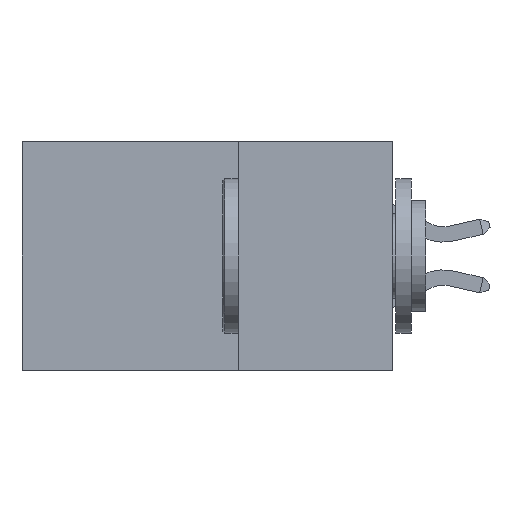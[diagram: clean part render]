
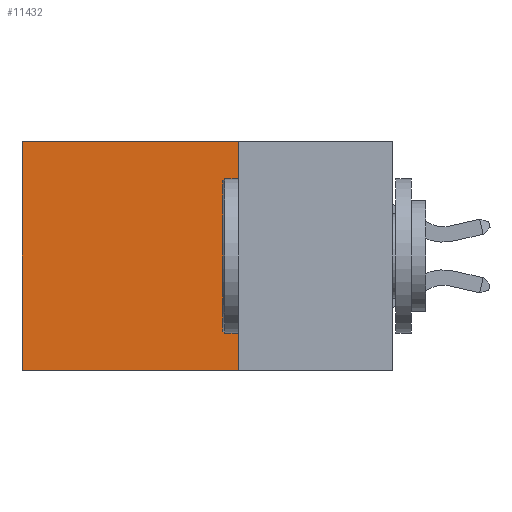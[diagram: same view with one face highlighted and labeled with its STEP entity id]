
A CAD part, left-side view. The second image highlights one B-rep face of the part: STEP entity #11432.
In plain terms, the highlighted planar face has unit normal (-1, 0, 0).
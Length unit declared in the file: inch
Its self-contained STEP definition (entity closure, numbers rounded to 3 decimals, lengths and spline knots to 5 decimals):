
#77 = AXIS2_PLACEMENT_3D ( 'NONE', #11838, #18074, #5435 ) ;
#2755 = VECTOR ( 'NONE', #4926, 39.37008 ) ;
#2768 = CARTESIAN_POINT ( 'NONE',  ( 0.2875, 0.25, -0.37 ) ) ;
#4536 = ORIENTED_EDGE ( 'NONE', *, *, #21344, .F. ) ;
#4926 = DIRECTION ( 'NONE',  ( 0., 0., -1. ) ) ;
#4946 = CARTESIAN_POINT ( 'NONE',  ( 0.2875, 0.6, -0.37 ) ) ;
#5435 = DIRECTION ( 'NONE',  ( 0., 0., -1. ) ) ;
#6113 = VECTOR ( 'NONE', #25194, 39.37008 ) ;
#6768 = LINE ( 'NONE', #23016, #6113 ) ;
#7376 = CARTESIAN_POINT ( 'NONE',  ( 0.2875, 0.25, 0. ) ) ;
#7511 = PLANE ( 'NONE',  #77 ) ;
#8352 = VERTEX_POINT ( 'NONE', #4946 ) ;
#8632 = LINE ( 'NONE', #7376, #19130 ) ;
#8957 = VERTEX_POINT ( 'NONE', #21779 ) ;
#9541 = DIRECTION ( 'NONE',  ( 0., 1., 0. ) ) ;
#11217 = FACE_OUTER_BOUND ( 'NONE', #12395, .T. ) ;
#11432 = ADVANCED_FACE ( 'NONE', ( #11217 ), #7511, .F. ) ;
#11838 = CARTESIAN_POINT ( 'NONE',  ( 0.2875, 0.25, 0. ) ) ;
#12133 = ORIENTED_EDGE ( 'NONE', *, *, #21604, .F. ) ;
#12395 = EDGE_LOOP ( 'NONE', ( #16885, #12133, #4536, #24022 ) ) ;
#13562 = LINE ( 'NONE', #19668, #2755 ) ;
#14515 = CARTESIAN_POINT ( 'NONE',  ( 0.2875, 0.25, -0.37 ) ) ;
#16806 = CARTESIAN_POINT ( 'NONE',  ( 0.2875, 0.6, 0. ) ) ;
#16885 = ORIENTED_EDGE ( 'NONE', *, *, #18298, .T. ) ;
#18074 = DIRECTION ( 'NONE',  ( 1., 0., 0. ) ) ;
#18075 = LINE ( 'NONE', #14515, #22937 ) ;
#18298 = EDGE_CURVE ( 'NONE', #21108, #8352, #6768, .T. ) ;
#19130 = VECTOR ( 'NONE', #9541, 39.37008 ) ;
#19499 = VERTEX_POINT ( 'NONE', #2768 ) ;
#19668 = CARTESIAN_POINT ( 'NONE',  ( 0.2875, 0.25, 0. ) ) ;
#20658 = DIRECTION ( 'NONE',  ( 0., 1., 0. ) ) ;
#21108 = VERTEX_POINT ( 'NONE', #16806 ) ;
#21344 = EDGE_CURVE ( 'NONE', #8957, #19499, #13562, .T. ) ;
#21604 = EDGE_CURVE ( 'NONE', #19499, #8352, #18075, .T. ) ;
#21779 = CARTESIAN_POINT ( 'NONE',  ( 0.2875, 0.25, 0. ) ) ;
#22937 = VECTOR ( 'NONE', #20658, 39.37008 ) ;
#23016 = CARTESIAN_POINT ( 'NONE',  ( 0.2875, 0.6, 0. ) ) ;
#24022 = ORIENTED_EDGE ( 'NONE', *, *, #26004, .T. ) ;
#25194 = DIRECTION ( 'NONE',  ( 0., 0., -1. ) ) ;
#26004 = EDGE_CURVE ( 'NONE', #8957, #21108, #8632, .T. ) ;
